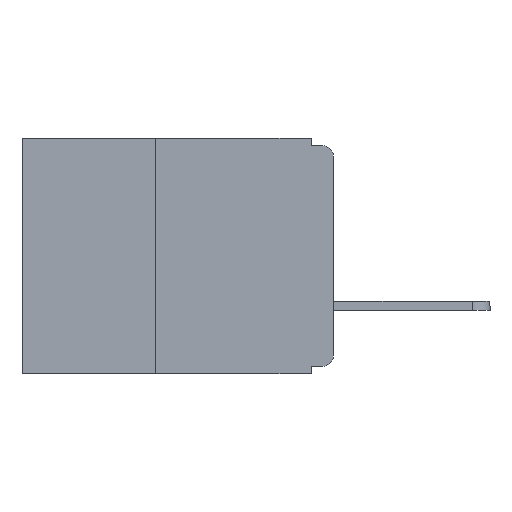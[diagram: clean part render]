
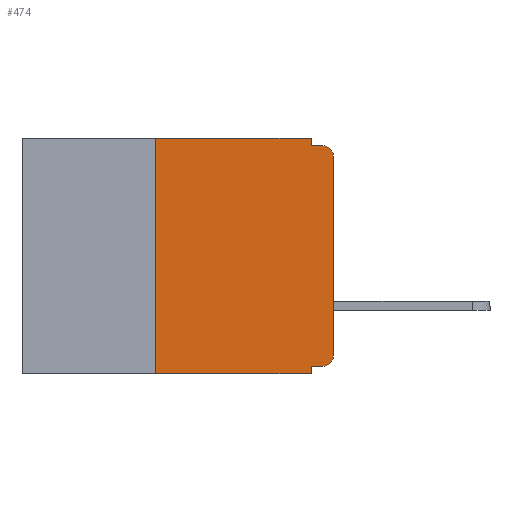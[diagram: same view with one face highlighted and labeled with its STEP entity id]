
A CAD part, left-side view. The second image highlights one B-rep face of the part: STEP entity #474.
In plain terms, the highlighted planar face has unit normal (-1, 0, 0).
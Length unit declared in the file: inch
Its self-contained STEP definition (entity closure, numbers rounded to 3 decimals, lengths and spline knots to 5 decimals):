
#269 = DIRECTION ( 'NONE',  ( -1., 0., 0. ) ) ;
#424 = LINE ( 'NONE', #18113, #4301 ) ;
#474 = ADVANCED_FACE ( 'NONE', ( #1952 ), #19736, .F. ) ;
#686 = EDGE_CURVE ( 'NONE', #1698, #22760, #6729, .T. ) ;
#720 = CARTESIAN_POINT ( 'NONE',  ( 0., 0., -0.025 ) ) ;
#957 = ORIENTED_EDGE ( 'NONE', *, *, #1469, .F. ) ;
#1210 = VERTEX_POINT ( 'NONE', #3150 ) ;
#1270 = DIRECTION ( 'NONE',  ( 0., 0., -1. ) ) ;
#1459 = CARTESIAN_POINT ( 'NONE',  ( 0., 0.015, -0.025 ) ) ;
#1469 = EDGE_CURVE ( 'NONE', #5962, #1210, #9042, .T. ) ;
#1698 = VERTEX_POINT ( 'NONE', #10096 ) ;
#1951 = CARTESIAN_POINT ( 'NONE',  ( 0., 0.015, -0.01 ) ) ;
#1952 = FACE_OUTER_BOUND ( 'NONE', #19992, .T. ) ;
#1960 = EDGE_CURVE ( 'NONE', #7028, #11066, #14681, .T. ) ;
#2005 = EDGE_CURVE ( 'NONE', #22760, #23146, #4048, .T. ) ;
#2225 = DIRECTION ( 'NONE',  ( 0., 0., -1. ) ) ;
#2226 = VERTEX_POINT ( 'NONE', #14515 ) ;
#2510 = LINE ( 'NONE', #10618, #16972 ) ;
#3092 = CARTESIAN_POINT ( 'NONE',  ( 0., 0.015, -0.305 ) ) ;
#3150 = CARTESIAN_POINT ( 'NONE',  ( 0., 0.031, -0.32 ) ) ;
#3226 = VECTOR ( 'NONE', #2225, 39.37008 ) ;
#3662 = CARTESIAN_POINT ( 'NONE',  ( 0., 0.031, -0.01 ) ) ;
#3992 = VECTOR ( 'NONE', #24212, 39.37008 ) ;
#4048 = CIRCLE ( 'NONE', #19926, 0.015 ) ;
#4301 = VECTOR ( 'NONE', #21942, 39.37008 ) ;
#4463 = ORIENTED_EDGE ( 'NONE', *, *, #20475, .F. ) ;
#4492 = EDGE_CURVE ( 'NONE', #5962, #1698, #11940, .T. ) ;
#5020 = ORIENTED_EDGE ( 'NONE', *, *, #686, .T. ) ;
#5033 = DIRECTION ( 'NONE',  ( 0., 0., -1. ) ) ;
#5269 = CARTESIAN_POINT ( 'NONE',  ( 0., 0.25, -0.33 ) ) ;
#5703 = VECTOR ( 'NONE', #21454, 39.37008 ) ;
#5962 = VERTEX_POINT ( 'NONE', #24567 ) ;
#6729 = LINE ( 'NONE', #15292, #16115 ) ;
#6909 = CARTESIAN_POINT ( 'NONE',  ( 0., 0.031, -0.33 ) ) ;
#7027 = DIRECTION ( 'NONE',  ( 0., -1., 0. ) ) ;
#7028 = VERTEX_POINT ( 'NONE', #5269 ) ;
#7656 = ORIENTED_EDGE ( 'NONE', *, *, #21505, .F. ) ;
#8077 = CARTESIAN_POINT ( 'NONE',  ( 0., 0.437, -0.33 ) ) ;
#8270 = CARTESIAN_POINT ( 'NONE',  ( 0., 0., -0.01 ) ) ;
#8724 = DIRECTION ( 'NONE',  ( 0., 0., -1. ) ) ;
#9042 = LINE ( 'NONE', #14777, #3992 ) ;
#9183 = ORIENTED_EDGE ( 'NONE', *, *, #1960, .T. ) ;
#9899 = LINE ( 'NONE', #16002, #24406 ) ;
#10096 = CARTESIAN_POINT ( 'NONE',  ( 0., 0., -0.305 ) ) ;
#10618 = CARTESIAN_POINT ( 'NONE',  ( 0., 0.031, -0.33 ) ) ;
#10665 = ORIENTED_EDGE ( 'NONE', *, *, #11051, .F. ) ;
#10722 = LINE ( 'NONE', #8270, #5703 ) ;
#11051 = EDGE_CURVE ( 'NONE', #1210, #11066, #2510, .T. ) ;
#11066 = VERTEX_POINT ( 'NONE', #6909 ) ;
#11940 = CIRCLE ( 'NONE', #16410, 0.015 ) ;
#11951 = CARTESIAN_POINT ( 'NONE',  ( 0., 0.25, 0. ) ) ;
#12565 = VERTEX_POINT ( 'NONE', #11951 ) ;
#12728 = LINE ( 'NONE', #15441, #3226 ) ;
#13874 = ORIENTED_EDGE ( 'NONE', *, *, #15671, .F. ) ;
#14227 = DIRECTION ( 'NONE',  ( 0., 0., 1. ) ) ;
#14515 = CARTESIAN_POINT ( 'NONE',  ( 0., 0.031, 0. ) ) ;
#14681 = LINE ( 'NONE', #8077, #24188 ) ;
#14777 = CARTESIAN_POINT ( 'NONE',  ( 0., 0., -0.32 ) ) ;
#15292 = CARTESIAN_POINT ( 'NONE',  ( 0., 0., 0. ) ) ;
#15441 = CARTESIAN_POINT ( 'NONE',  ( 0., 0.031, 0. ) ) ;
#15657 = DIRECTION ( 'NONE',  ( 0., 0., 1. ) ) ;
#15671 = EDGE_CURVE ( 'NONE', #2226, #17271, #12728, .T. ) ;
#16002 = CARTESIAN_POINT ( 'NONE',  ( 0., 0.25, -0.33 ) ) ;
#16115 = VECTOR ( 'NONE', #15657, 39.37008 ) ;
#16287 = DIRECTION ( 'NONE',  ( -1., 0., 0. ) ) ;
#16410 = AXIS2_PLACEMENT_3D ( 'NONE', #3092, #16287, #5033 ) ;
#16972 = VECTOR ( 'NONE', #8724, 39.37008 ) ;
#17271 = VERTEX_POINT ( 'NONE', #3662 ) ;
#17979 = ORIENTED_EDGE ( 'NONE', *, *, #18150, .F. ) ;
#18113 = CARTESIAN_POINT ( 'NONE',  ( 0., 0.437, 0. ) ) ;
#18150 = EDGE_CURVE ( 'NONE', #12565, #2226, #424, .T. ) ;
#19736 = PLANE ( 'NONE',  #20999 ) ;
#19765 = CARTESIAN_POINT ( 'NONE',  ( 0., 0.437, 0. ) ) ;
#19892 = ORIENTED_EDGE ( 'NONE', *, *, #4492, .T. ) ;
#19926 = AXIS2_PLACEMENT_3D ( 'NONE', #1459, #269, #1270 ) ;
#19992 = EDGE_LOOP ( 'NONE', ( #5020, #24443, #7656, #13874, #17979, #4463, #9183, #10665, #957, #19892 ) ) ;
#20475 = EDGE_CURVE ( 'NONE', #7028, #12565, #9899, .T. ) ;
#20999 = AXIS2_PLACEMENT_3D ( 'NONE', #19765, #22286, #22924 ) ;
#21454 = DIRECTION ( 'NONE',  ( 0., -1., 0. ) ) ;
#21505 = EDGE_CURVE ( 'NONE', #17271, #23146, #10722, .T. ) ;
#21942 = DIRECTION ( 'NONE',  ( 0., -1., 0. ) ) ;
#22286 = DIRECTION ( 'NONE',  ( 1., 0., 0. ) ) ;
#22760 = VERTEX_POINT ( 'NONE', #720 ) ;
#22924 = DIRECTION ( 'NONE',  ( 0., 0., -1. ) ) ;
#23146 = VERTEX_POINT ( 'NONE', #1951 ) ;
#24188 = VECTOR ( 'NONE', #7027, 39.37008 ) ;
#24212 = DIRECTION ( 'NONE',  ( 0., 1., 0. ) ) ;
#24406 = VECTOR ( 'NONE', #14227, 39.37008 ) ;
#24443 = ORIENTED_EDGE ( 'NONE', *, *, #2005, .T. ) ;
#24567 = CARTESIAN_POINT ( 'NONE',  ( 0., 0.015, -0.32 ) ) ;
